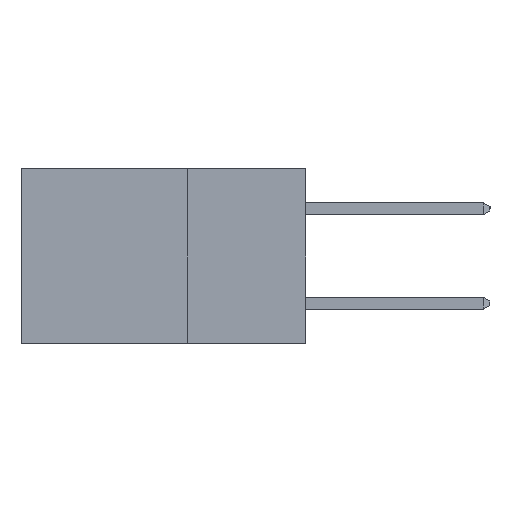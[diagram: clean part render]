
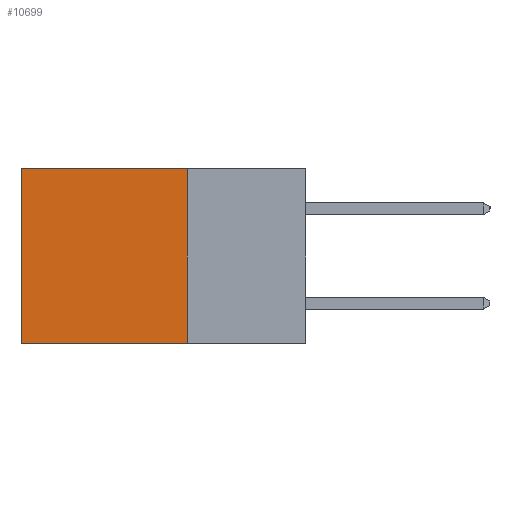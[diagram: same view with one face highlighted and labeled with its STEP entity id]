
A CAD part, left-side view. The second image highlights one B-rep face of the part: STEP entity #10699.
In plain terms, the highlighted planar face has unit normal (-1, 0, 0).
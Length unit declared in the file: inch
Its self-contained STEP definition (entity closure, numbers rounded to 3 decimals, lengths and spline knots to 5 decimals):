
#894 = CARTESIAN_POINT ( 'NONE',  ( 0.2615, 0.25, 0. ) ) ;
#1543 = EDGE_CURVE ( 'NONE', #8644, #10587, #5510, .T. ) ;
#1857 = LINE ( 'NONE', #2902, #11367 ) ;
#1907 = EDGE_CURVE ( 'NONE', #2649, #3377, #4663, .T. ) ;
#2649 = VERTEX_POINT ( 'NONE', #11634 ) ;
#2902 = CARTESIAN_POINT ( 'NONE',  ( 0.2615, 0.25, -0.37 ) ) ;
#3287 = AXIS2_PLACEMENT_3D ( 'NONE', #3390, #7943, #4288 ) ;
#3333 = PLANE ( 'NONE',  #3287 ) ;
#3377 = VERTEX_POINT ( 'NONE', #4041 ) ;
#3390 = CARTESIAN_POINT ( 'NONE',  ( 0.2615, 0.25, -0.37 ) ) ;
#3716 = DIRECTION ( 'NONE',  ( 0., 0., -1. ) ) ;
#3911 = CARTESIAN_POINT ( 'NONE',  ( 0.2615, 0.25, -0.37 ) ) ;
#4041 = CARTESIAN_POINT ( 'NONE',  ( 0.2615, 0.6, -0.37 ) ) ;
#4288 = DIRECTION ( 'NONE',  ( 0., 0., -1. ) ) ;
#4343 = FACE_OUTER_BOUND ( 'NONE', #10885, .T. ) ;
#4513 = DIRECTION ( 'NONE',  ( 0., 1., 0. ) ) ;
#4663 = LINE ( 'NONE', #8265, #5047 ) ;
#4883 = ORIENTED_EDGE ( 'NONE', *, *, #10474, .F. ) ;
#5047 = VECTOR ( 'NONE', #3716, 39.37008 ) ;
#5510 = LINE ( 'NONE', #10862, #6724 ) ;
#6483 = VECTOR ( 'NONE', #4513, 39.37008 ) ;
#6724 = VECTOR ( 'NONE', #7541, 39.37008 ) ;
#7541 = DIRECTION ( 'NONE',  ( 0., 0., -1. ) ) ;
#7646 = ORIENTED_EDGE ( 'NONE', *, *, #10930, .T. ) ;
#7688 = CARTESIAN_POINT ( 'NONE',  ( 0.2615, 0.25, 0. ) ) ;
#7943 = DIRECTION ( 'NONE',  ( 1., 0., 0. ) ) ;
#8265 = CARTESIAN_POINT ( 'NONE',  ( 0.2615, 0.6, -0.37 ) ) ;
#8278 = ORIENTED_EDGE ( 'NONE', *, *, #1907, .T. ) ;
#8644 = VERTEX_POINT ( 'NONE', #7688 ) ;
#9004 = LINE ( 'NONE', #894, #6483 ) ;
#9063 = DIRECTION ( 'NONE',  ( 0., 1., 0. ) ) ;
#9792 = ORIENTED_EDGE ( 'NONE', *, *, #1543, .F. ) ;
#10474 = EDGE_CURVE ( 'NONE', #10587, #3377, #1857, .T. ) ;
#10587 = VERTEX_POINT ( 'NONE', #3911 ) ;
#10699 = ADVANCED_FACE ( 'NONE', ( #4343 ), #3333, .F. ) ;
#10862 = CARTESIAN_POINT ( 'NONE',  ( 0.2615, 0.25, -0.37 ) ) ;
#10885 = EDGE_LOOP ( 'NONE', ( #8278, #4883, #9792, #7646 ) ) ;
#10930 = EDGE_CURVE ( 'NONE', #8644, #2649, #9004, .T. ) ;
#11367 = VECTOR ( 'NONE', #9063, 39.37008 ) ;
#11634 = CARTESIAN_POINT ( 'NONE',  ( 0.2615, 0.6, 0. ) ) ;
